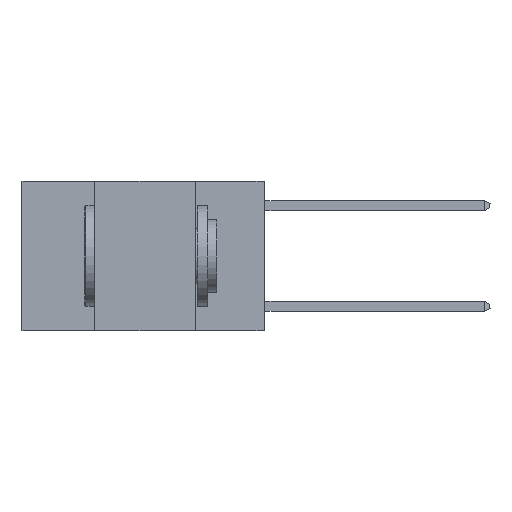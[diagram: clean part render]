
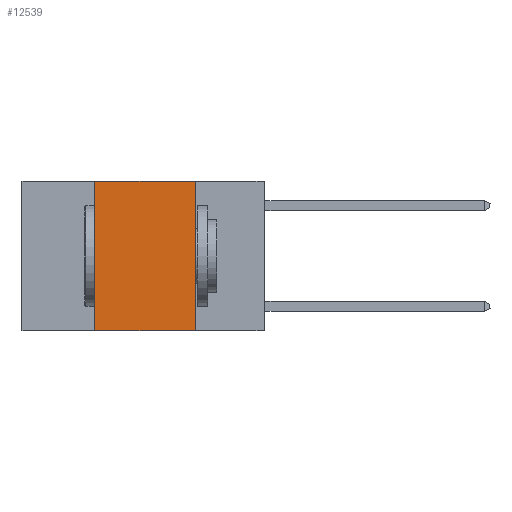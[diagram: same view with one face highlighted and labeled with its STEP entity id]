
A CAD part, left-side view. The second image highlights one B-rep face of the part: STEP entity #12539.
In plain terms, the highlighted planar face has unit normal (-1, 0, 0).
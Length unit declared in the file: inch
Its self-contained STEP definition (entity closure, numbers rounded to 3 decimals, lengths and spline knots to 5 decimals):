
#220 = AXIS2_PLACEMENT_3D ( 'NONE', #960, #2196, #15987 ) ;
#354 = ORIENTED_EDGE ( 'NONE', *, *, #1204, .T. ) ;
#711 = PLANE ( 'NONE',  #220 ) ;
#960 = CARTESIAN_POINT ( 'NONE',  ( 0., 0.6, 0. ) ) ;
#1204 = EDGE_CURVE ( 'NONE', #5252, #4994, #13678, .T. ) ;
#2063 = CARTESIAN_POINT ( 'NONE',  ( 0., 0.17, -0.37 ) ) ;
#2080 = VECTOR ( 'NONE', #3778, 39.37008 ) ;
#2196 = DIRECTION ( 'NONE',  ( 1., 0., 0. ) ) ;
#2257 = DIRECTION ( 'NONE',  ( 0., -1., 0. ) ) ;
#3778 = DIRECTION ( 'NONE',  ( 0., -1., 0. ) ) ;
#4185 = CARTESIAN_POINT ( 'NONE',  ( 0., 0.42, 0. ) ) ;
#4769 = CARTESIAN_POINT ( 'NONE',  ( 0., 0.42, 0. ) ) ;
#4926 = CARTESIAN_POINT ( 'NONE',  ( 0., 0.42, -0.37 ) ) ;
#4994 = VERTEX_POINT ( 'NONE', #2063 ) ;
#5252 = VERTEX_POINT ( 'NONE', #4926 ) ;
#5254 = ORIENTED_EDGE ( 'NONE', *, *, #15344, .F. ) ;
#5355 = EDGE_CURVE ( 'NONE', #5252, #11177, #14223, .T. ) ;
#6648 = EDGE_CURVE ( 'NONE', #7043, #4994, #7985, .T. ) ;
#7043 = VERTEX_POINT ( 'NONE', #13958 ) ;
#7307 = FACE_OUTER_BOUND ( 'NONE', #11354, .T. ) ;
#7493 = CARTESIAN_POINT ( 'NONE',  ( 0., 0.6, 0. ) ) ;
#7624 = ORIENTED_EDGE ( 'NONE', *, *, #5355, .F. ) ;
#7735 = DIRECTION ( 'NONE',  ( 0., 0., 1. ) ) ;
#7985 = LINE ( 'NONE', #11686, #15171 ) ;
#8494 = LINE ( 'NONE', #7493, #2080 ) ;
#10463 = DIRECTION ( 'NONE',  ( 0., 0., -1. ) ) ;
#10692 = VECTOR ( 'NONE', #7735, 39.37008 ) ;
#11177 = VERTEX_POINT ( 'NONE', #4769 ) ;
#11354 = EDGE_LOOP ( 'NONE', ( #13321, #5254, #7624, #354 ) ) ;
#11686 = CARTESIAN_POINT ( 'NONE',  ( 0., 0.17, 0. ) ) ;
#12297 = CARTESIAN_POINT ( 'NONE',  ( 0., 0.6, -0.37 ) ) ;
#12539 = ADVANCED_FACE ( 'NONE', ( #7307 ), #711, .F. ) ;
#12661 = VECTOR ( 'NONE', #2257, 39.37008 ) ;
#13321 = ORIENTED_EDGE ( 'NONE', *, *, #6648, .F. ) ;
#13678 = LINE ( 'NONE', #12297, #12661 ) ;
#13958 = CARTESIAN_POINT ( 'NONE',  ( 0., 0.17, 0. ) ) ;
#14223 = LINE ( 'NONE', #4185, #10692 ) ;
#15171 = VECTOR ( 'NONE', #10463, 39.37008 ) ;
#15344 = EDGE_CURVE ( 'NONE', #11177, #7043, #8494, .T. ) ;
#15987 = DIRECTION ( 'NONE',  ( 0., 0., -1. ) ) ;
